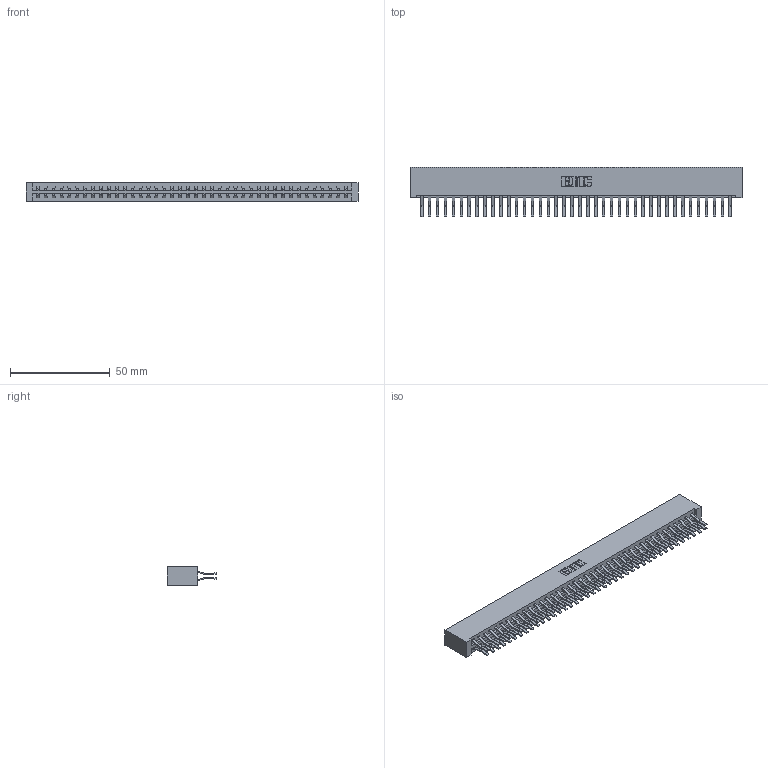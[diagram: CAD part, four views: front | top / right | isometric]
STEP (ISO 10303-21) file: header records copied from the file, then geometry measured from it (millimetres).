
FILE_DESCRIPTION (( 'STEP AP203' ), '1' );
FILE_NAME ('337-080-560-201.STEP', '2018-08-12T19:09:19', ( '' ), ( '' ), 'SwSTEP 2.0', 'SolidWorks 2016', '' );
FILE_SCHEMA (( 'CONFIG_CONTROL_DESIGN' ));
Length unit declared in the file: inch
Products named in the file (3): 337 Part_No Mounting Lugs; 345-292-001_560 Tail; 337-080-560-201
Assembly tree (81 placements, depth 2):
  337-080-560-201
    337 Part_No Mounting Lugs
    345-292-001_560 Tail  x80
Bounding box: 166.37 x 24.78 x 9.4 mm (x, y, z)
Volume: 18791.9 mm3; surface area: 22798.6 mm2
Topology: 81 solids, 81 shells, 4586 faces, 13647 edges, 8990 vertices
Faces by surface type: plane 3106, cylinder 1480
Entity records: 31083 total; most frequent: CARTESIAN_POINT 5238, ORIENTED_EDGE 5174, DIRECTION 4455, EDGE_CURVE 2587, LINE 2463, VECTOR 2463, VERTEX_POINT 1722, AXIS2_PLACEMENT_3D 996
